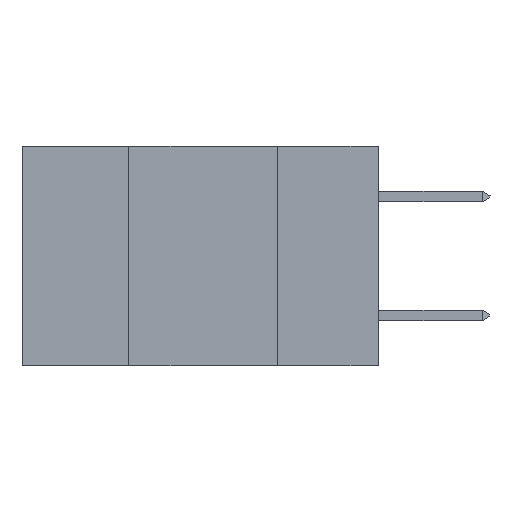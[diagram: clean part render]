
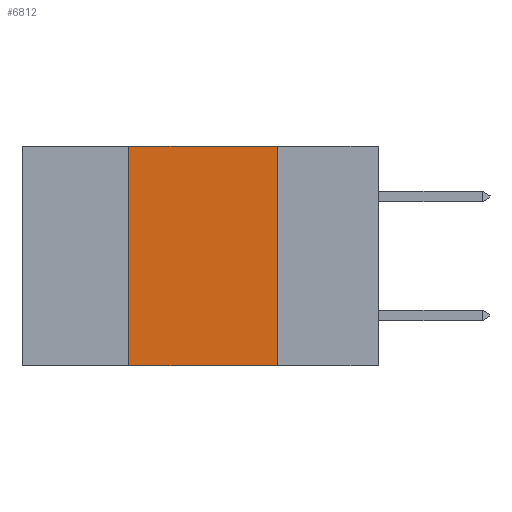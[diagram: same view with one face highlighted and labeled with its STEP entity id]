
A CAD part, left-side view. The second image highlights one B-rep face of the part: STEP entity #6812.
In plain terms, the highlighted planar face has unit normal (-1, 0, 0).
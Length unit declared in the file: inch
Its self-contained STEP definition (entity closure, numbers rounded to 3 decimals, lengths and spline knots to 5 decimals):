
#1317 = DIRECTION ( 'NONE',  ( 0., -1., 0. ) ) ;
#1557 = EDGE_CURVE ( 'NONE', #2161, #16325, #4360, .T. ) ;
#1660 = VERTEX_POINT ( 'NONE', #6661 ) ;
#2161 = VERTEX_POINT ( 'NONE', #10080 ) ;
#2836 = EDGE_CURVE ( 'NONE', #1660, #18541, #8499, .T. ) ;
#3075 = VECTOR ( 'NONE', #12128, 39.37008 ) ;
#4360 = LINE ( 'NONE', #16195, #15064 ) ;
#4977 = ORIENTED_EDGE ( 'NONE', *, *, #2836, .F. ) ;
#6138 = DIRECTION ( 'NONE',  ( 1., 0., 0. ) ) ;
#6661 = CARTESIAN_POINT ( 'NONE',  ( 0., 0.17, 0. ) ) ;
#6812 = ADVANCED_FACE ( 'NONE', ( #20064 ), #15070, .F. ) ;
#7284 = LINE ( 'NONE', #20900, #13702 ) ;
#8499 = LINE ( 'NONE', #16897, #3075 ) ;
#9477 = CARTESIAN_POINT ( 'NONE',  ( 0., 0.42, 0. ) ) ;
#9556 = ORIENTED_EDGE ( 'NONE', *, *, #13497, .F. ) ;
#9668 = DIRECTION ( 'NONE',  ( 0., 0., -1. ) ) ;
#9698 = AXIS2_PLACEMENT_3D ( 'NONE', #12978, #6138, #9668 ) ;
#9703 = LINE ( 'NONE', #16443, #19615 ) ;
#10080 = CARTESIAN_POINT ( 'NONE',  ( 0., 0.42, -0.37 ) ) ;
#10766 = ORIENTED_EDGE ( 'NONE', *, *, #18371, .T. ) ;
#11490 = EDGE_LOOP ( 'NONE', ( #4977, #9556, #19146, #10766 ) ) ;
#12128 = DIRECTION ( 'NONE',  ( 0., 0., -1. ) ) ;
#12162 = DIRECTION ( 'NONE',  ( 0., -1., 0. ) ) ;
#12978 = CARTESIAN_POINT ( 'NONE',  ( 0., 0.6, 0. ) ) ;
#13497 = EDGE_CURVE ( 'NONE', #16325, #1660, #7284, .T. ) ;
#13702 = VECTOR ( 'NONE', #12162, 39.37008 ) ;
#14519 = DIRECTION ( 'NONE',  ( 0., 0., 1. ) ) ;
#15064 = VECTOR ( 'NONE', #14519, 39.37008 ) ;
#15070 = PLANE ( 'NONE',  #9698 ) ;
#16195 = CARTESIAN_POINT ( 'NONE',  ( 0., 0.42, -0.37 ) ) ;
#16325 = VERTEX_POINT ( 'NONE', #9477 ) ;
#16443 = CARTESIAN_POINT ( 'NONE',  ( 0., 0.6, -0.37 ) ) ;
#16897 = CARTESIAN_POINT ( 'NONE',  ( 0., 0.17, -0.37 ) ) ;
#17422 = CARTESIAN_POINT ( 'NONE',  ( 0., 0.17, -0.37 ) ) ;
#18371 = EDGE_CURVE ( 'NONE', #2161, #18541, #9703, .T. ) ;
#18541 = VERTEX_POINT ( 'NONE', #17422 ) ;
#19146 = ORIENTED_EDGE ( 'NONE', *, *, #1557, .F. ) ;
#19615 = VECTOR ( 'NONE', #1317, 39.37008 ) ;
#20064 = FACE_OUTER_BOUND ( 'NONE', #11490, .T. ) ;
#20900 = CARTESIAN_POINT ( 'NONE',  ( 0., 0.6, 0. ) ) ;
